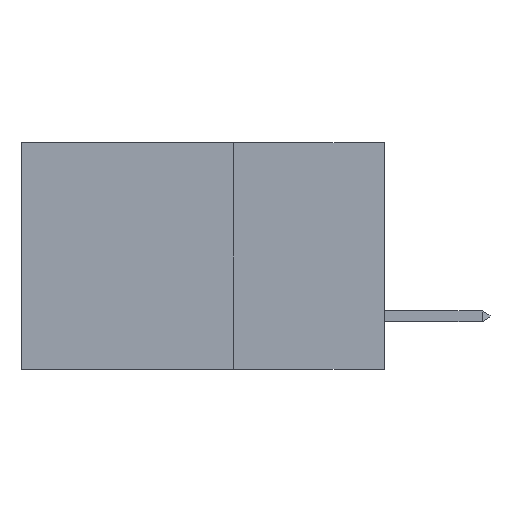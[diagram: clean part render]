
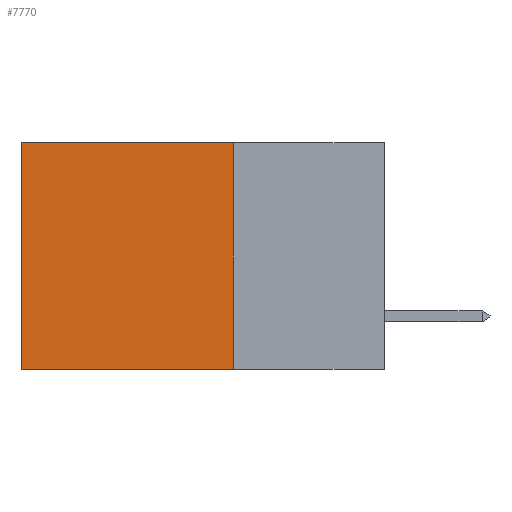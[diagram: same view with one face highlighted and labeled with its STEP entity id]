
A CAD part, left-side view. The second image highlights one B-rep face of the part: STEP entity #7770.
In plain terms, the highlighted planar face has unit normal (-1, 0, 0).
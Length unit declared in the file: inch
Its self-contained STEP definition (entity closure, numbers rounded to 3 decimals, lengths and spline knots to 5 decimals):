
#163 = VERTEX_POINT ( 'NONE', #2119 ) ;
#698 = ORIENTED_EDGE ( 'NONE', *, *, #1777, .F. ) ;
#787 = LINE ( 'NONE', #6036, #8130 ) ;
#1777 = EDGE_CURVE ( 'NONE', #6150, #5665, #3419, .T. ) ;
#2013 = DIRECTION ( 'NONE',  ( 0., 0., -1. ) ) ;
#2119 = CARTESIAN_POINT ( 'NONE',  ( 0.2875, 0.25, 0. ) ) ;
#2484 = VECTOR ( 'NONE', #4415, 39.37008 ) ;
#2727 = FACE_OUTER_BOUND ( 'NONE', #8435, .T. ) ;
#2733 = VECTOR ( 'NONE', #6432, 39.37008 ) ;
#2864 = ORIENTED_EDGE ( 'NONE', *, *, #4938, .F. ) ;
#3157 = EDGE_CURVE ( 'NONE', #163, #6137, #3238, .T. ) ;
#3207 = CARTESIAN_POINT ( 'NONE',  ( 0.2875, 0.6, -0.375 ) ) ;
#3238 = LINE ( 'NONE', #3904, #2733 ) ;
#3419 = LINE ( 'NONE', #6866, #5790 ) ;
#3433 = CARTESIAN_POINT ( 'NONE',  ( 0.2875, 0.25, -0.375 ) ) ;
#3904 = CARTESIAN_POINT ( 'NONE',  ( 0.2875, 0.25, 0. ) ) ;
#4220 = ORIENTED_EDGE ( 'NONE', *, *, #3157, .T. ) ;
#4226 = DIRECTION ( 'NONE',  ( 0., 1., 0. ) ) ;
#4415 = DIRECTION ( 'NONE',  ( 0., 0., -1. ) ) ;
#4938 = EDGE_CURVE ( 'NONE', #163, #6150, #7352, .T. ) ;
#5562 = CARTESIAN_POINT ( 'NONE',  ( 0.2875, 0.25, -0.375 ) ) ;
#5665 = VERTEX_POINT ( 'NONE', #3207 ) ;
#5790 = VECTOR ( 'NONE', #4226, 39.37008 ) ;
#5957 = DIRECTION ( 'NONE',  ( 1., 0., 0. ) ) ;
#6006 = AXIS2_PLACEMENT_3D ( 'NONE', #7876, #5957, #2013 ) ;
#6036 = CARTESIAN_POINT ( 'NONE',  ( 0.2875, 0.6, -0.375 ) ) ;
#6065 = CARTESIAN_POINT ( 'NONE',  ( 0.2875, 0.6, 0. ) ) ;
#6137 = VERTEX_POINT ( 'NONE', #6065 ) ;
#6150 = VERTEX_POINT ( 'NONE', #3433 ) ;
#6432 = DIRECTION ( 'NONE',  ( 0., 1., 0. ) ) ;
#6866 = CARTESIAN_POINT ( 'NONE',  ( 0.2875, 0.25, -0.375 ) ) ;
#7352 = LINE ( 'NONE', #5562, #2484 ) ;
#7766 = PLANE ( 'NONE',  #6006 ) ;
#7770 = ADVANCED_FACE ( 'NONE', ( #2727 ), #7766, .F. ) ;
#7876 = CARTESIAN_POINT ( 'NONE',  ( 0.2875, 0.25, -0.375 ) ) ;
#7883 = EDGE_CURVE ( 'NONE', #6137, #5665, #787, .T. ) ;
#8010 = DIRECTION ( 'NONE',  ( 0., 0., -1. ) ) ;
#8029 = ORIENTED_EDGE ( 'NONE', *, *, #7883, .T. ) ;
#8130 = VECTOR ( 'NONE', #8010, 39.37008 ) ;
#8435 = EDGE_LOOP ( 'NONE', ( #8029, #698, #2864, #4220 ) ) ;
